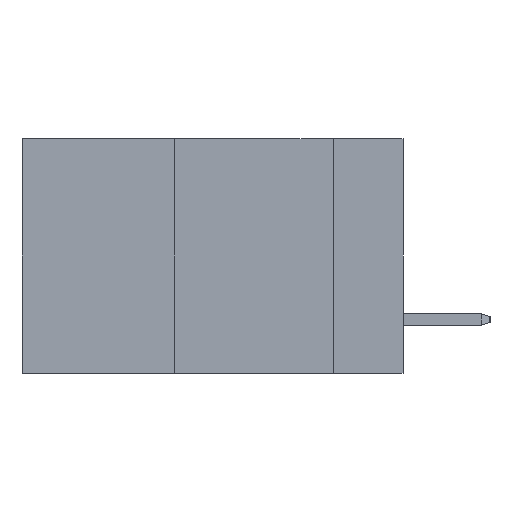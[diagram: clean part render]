
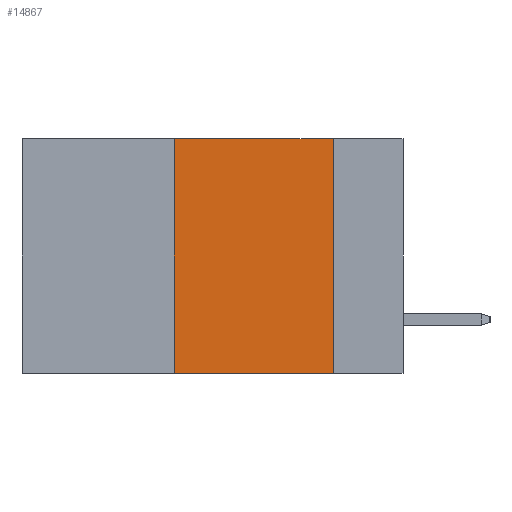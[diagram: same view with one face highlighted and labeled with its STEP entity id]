
A CAD part, left-side view. The second image highlights one B-rep face of the part: STEP entity #14867.
In plain terms, the highlighted planar face has unit normal (-1, 0, 0).
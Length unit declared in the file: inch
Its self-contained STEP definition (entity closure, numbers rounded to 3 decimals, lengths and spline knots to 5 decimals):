
#244 = VERTEX_POINT ( 'NONE', #2649 ) ;
#1623 = LINE ( 'NONE', #14876, #9460 ) ;
#1927 = VERTEX_POINT ( 'NONE', #4880 ) ;
#2649 = CARTESIAN_POINT ( 'NONE',  ( 0., 0.36, 0. ) ) ;
#2697 = DIRECTION ( 'NONE',  ( 0., 0., -1. ) ) ;
#2731 = DIRECTION ( 'NONE',  ( 0., -1., 0. ) ) ;
#2915 = ORIENTED_EDGE ( 'NONE', *, *, #8110, .T. ) ;
#4255 = CARTESIAN_POINT ( 'NONE',  ( 0., 0.6, 0. ) ) ;
#4306 = ORIENTED_EDGE ( 'NONE', *, *, #8134, .F. ) ;
#4557 = VERTEX_POINT ( 'NONE', #15420 ) ;
#4880 = CARTESIAN_POINT ( 'NONE',  ( 0., 0.11, -0.37 ) ) ;
#5716 = VECTOR ( 'NONE', #10576, 39.37008 ) ;
#5721 = LINE ( 'NONE', #15388, #5716 ) ;
#6274 = DIRECTION ( 'NONE',  ( 0., 0., 1. ) ) ;
#6414 = EDGE_LOOP ( 'NONE', ( #4306, #14016, #14709, #2915 ) ) ;
#6729 = DIRECTION ( 'NONE',  ( 1., 0., 0. ) ) ;
#7622 = CARTESIAN_POINT ( 'NONE',  ( 0., 0.36, 0. ) ) ;
#8110 = EDGE_CURVE ( 'NONE', #15702, #1927, #1623, .T. ) ;
#8134 = EDGE_CURVE ( 'NONE', #4557, #1927, #15726, .T. ) ;
#9460 = VECTOR ( 'NONE', #2731, 39.37008 ) ;
#9630 = EDGE_CURVE ( 'NONE', #15702, #244, #12171, .T. ) ;
#9647 = CARTESIAN_POINT ( 'NONE',  ( 0., 0.11, 0. ) ) ;
#10576 = DIRECTION ( 'NONE',  ( 0., -1., 0. ) ) ;
#10679 = VECTOR ( 'NONE', #6274, 39.37008 ) ;
#12171 = LINE ( 'NONE', #7622, #10679 ) ;
#12453 = EDGE_CURVE ( 'NONE', #244, #4557, #5721, .T. ) ;
#13409 = AXIS2_PLACEMENT_3D ( 'NONE', #4255, #6729, #2697 ) ;
#13629 = CARTESIAN_POINT ( 'NONE',  ( 0., 0.36, -0.37 ) ) ;
#13633 = FACE_OUTER_BOUND ( 'NONE', #6414, .T. ) ;
#14016 = ORIENTED_EDGE ( 'NONE', *, *, #12453, .F. ) ;
#14061 = VECTOR ( 'NONE', #14440, 39.37008 ) ;
#14440 = DIRECTION ( 'NONE',  ( 0., 0., -1. ) ) ;
#14709 = ORIENTED_EDGE ( 'NONE', *, *, #9630, .F. ) ;
#14867 = ADVANCED_FACE ( 'NONE', ( #13633 ), #14922, .F. ) ;
#14876 = CARTESIAN_POINT ( 'NONE',  ( 0., 0.6, -0.37 ) ) ;
#14922 = PLANE ( 'NONE',  #13409 ) ;
#15388 = CARTESIAN_POINT ( 'NONE',  ( 0., 0.6, 0. ) ) ;
#15420 = CARTESIAN_POINT ( 'NONE',  ( 0., 0.11, 0. ) ) ;
#15702 = VERTEX_POINT ( 'NONE', #13629 ) ;
#15726 = LINE ( 'NONE', #9647, #14061 ) ;
